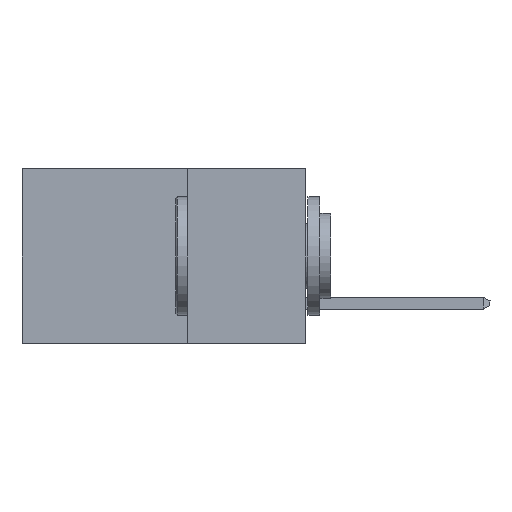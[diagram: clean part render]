
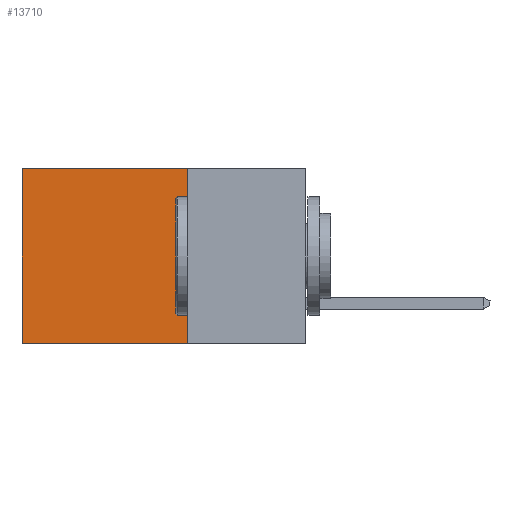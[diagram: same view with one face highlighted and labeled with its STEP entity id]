
A CAD part, left-side view. The second image highlights one B-rep face of the part: STEP entity #13710.
In plain terms, the highlighted planar face has unit normal (-1, 0, 0).
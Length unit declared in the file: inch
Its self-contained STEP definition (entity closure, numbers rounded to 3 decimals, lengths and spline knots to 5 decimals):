
#457 = DIRECTION ( 'NONE',  ( 0., 1., 0. ) ) ;
#467 = EDGE_CURVE ( 'NONE', #4553, #11020, #15070, .T. ) ;
#995 = DIRECTION ( 'NONE',  ( 0., 0., -1. ) ) ;
#1047 = LINE ( 'NONE', #18051, #14280 ) ;
#1524 = VECTOR ( 'NONE', #995, 39.37008 ) ;
#3159 = EDGE_CURVE ( 'NONE', #11020, #7949, #3858, .T. ) ;
#3200 = CARTESIAN_POINT ( 'NONE',  ( 0.2615, 0.25, -0.37 ) ) ;
#3858 = LINE ( 'NONE', #11586, #1524 ) ;
#3964 = CARTESIAN_POINT ( 'NONE',  ( 0.2615, 0.6, -0.37 ) ) ;
#4553 = VERTEX_POINT ( 'NONE', #7239 ) ;
#4649 = ORIENTED_EDGE ( 'NONE', *, *, #8216, .F. ) ;
#5248 = LINE ( 'NONE', #3200, #18246 ) ;
#5310 = DIRECTION ( 'NONE',  ( 1., 0., 0. ) ) ;
#5911 = EDGE_CURVE ( 'NONE', #4553, #10719, #1047, .T. ) ;
#6973 = AXIS2_PLACEMENT_3D ( 'NONE', #19229, #5310, #11506 ) ;
#7239 = CARTESIAN_POINT ( 'NONE',  ( 0.2615, 0.25, 0. ) ) ;
#7427 = ORIENTED_EDGE ( 'NONE', *, *, #5911, .F. ) ;
#7700 = VECTOR ( 'NONE', #12208, 39.37008 ) ;
#7949 = VERTEX_POINT ( 'NONE', #3964 ) ;
#8216 = EDGE_CURVE ( 'NONE', #10719, #7949, #5248, .T. ) ;
#9657 = ORIENTED_EDGE ( 'NONE', *, *, #467, .T. ) ;
#10719 = VERTEX_POINT ( 'NONE', #19200 ) ;
#11020 = VERTEX_POINT ( 'NONE', #18785 ) ;
#11506 = DIRECTION ( 'NONE',  ( 0., 0., -1. ) ) ;
#11586 = CARTESIAN_POINT ( 'NONE',  ( 0.2615, 0.6, -0.37 ) ) ;
#11607 = FACE_OUTER_BOUND ( 'NONE', #11937, .T. ) ;
#11937 = EDGE_LOOP ( 'NONE', ( #16873, #4649, #7427, #9657 ) ) ;
#11943 = DIRECTION ( 'NONE',  ( 0., 0., -1. ) ) ;
#12208 = DIRECTION ( 'NONE',  ( 0., 1., 0. ) ) ;
#13535 = CARTESIAN_POINT ( 'NONE',  ( 0.2615, 0.25, 0. ) ) ;
#13710 = ADVANCED_FACE ( 'NONE', ( #11607 ), #17803, .F. ) ;
#14280 = VECTOR ( 'NONE', #11943, 39.37008 ) ;
#15070 = LINE ( 'NONE', #13535, #7700 ) ;
#16873 = ORIENTED_EDGE ( 'NONE', *, *, #3159, .T. ) ;
#17803 = PLANE ( 'NONE',  #6973 ) ;
#18051 = CARTESIAN_POINT ( 'NONE',  ( 0.2615, 0.25, -0.37 ) ) ;
#18246 = VECTOR ( 'NONE', #457, 39.37008 ) ;
#18785 = CARTESIAN_POINT ( 'NONE',  ( 0.2615, 0.6, 0. ) ) ;
#19200 = CARTESIAN_POINT ( 'NONE',  ( 0.2615, 0.25, -0.37 ) ) ;
#19229 = CARTESIAN_POINT ( 'NONE',  ( 0.2615, 0.25, -0.37 ) ) ;
